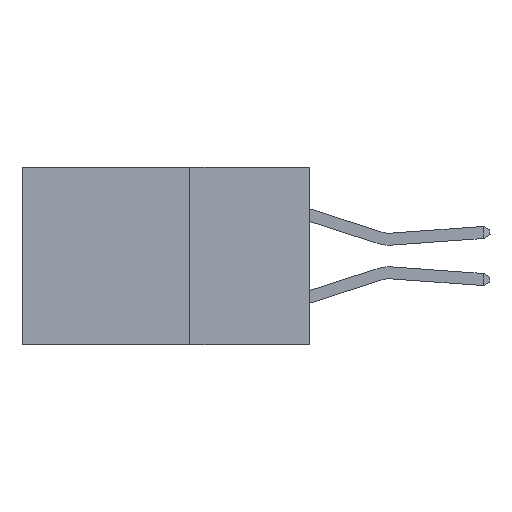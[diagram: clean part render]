
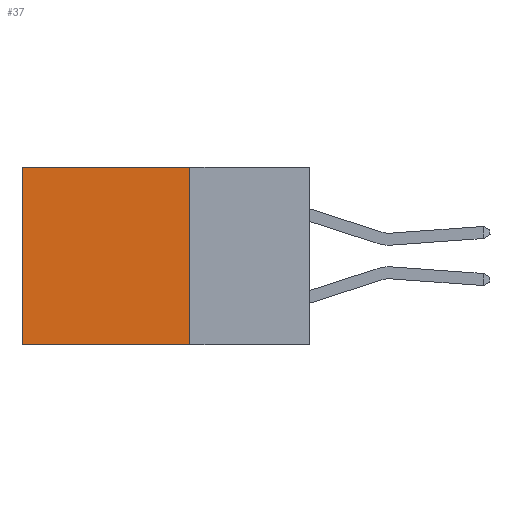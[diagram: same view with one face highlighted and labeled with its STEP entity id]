
A CAD part, left-side view. The second image highlights one B-rep face of the part: STEP entity #37.
In plain terms, the highlighted planar face has unit normal (-1, 0, 0).
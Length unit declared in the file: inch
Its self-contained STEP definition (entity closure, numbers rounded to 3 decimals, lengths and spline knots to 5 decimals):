
#37 = ADVANCED_FACE ( 'NONE', ( #2253 ), #18303, .F. ) ;
#833 = EDGE_LOOP ( 'NONE', ( #8648, #12536, #7388, #7956 ) ) ;
#2059 = LINE ( 'NONE', #13788, #10740 ) ;
#2253 = FACE_OUTER_BOUND ( 'NONE', #833, .T. ) ;
#3085 = DIRECTION ( 'NONE',  ( 0., 0., -1. ) ) ;
#3976 = DIRECTION ( 'NONE',  ( 0., 1., 0. ) ) ;
#4777 = VECTOR ( 'NONE', #19319, 39.37008 ) ;
#6428 = DIRECTION ( 'NONE',  ( 1., 0., 0. ) ) ;
#7052 = EDGE_CURVE ( 'NONE', #10376, #7203, #2059, .T. ) ;
#7203 = VERTEX_POINT ( 'NONE', #9195 ) ;
#7388 = ORIENTED_EDGE ( 'NONE', *, *, #11854, .F. ) ;
#7956 = ORIENTED_EDGE ( 'NONE', *, *, #20057, .T. ) ;
#7968 = DIRECTION ( 'NONE',  ( 0., 0., -1. ) ) ;
#8616 = LINE ( 'NONE', #16102, #16785 ) ;
#8648 = ORIENTED_EDGE ( 'NONE', *, *, #20054, .T. ) ;
#8973 = AXIS2_PLACEMENT_3D ( 'NONE', #20488, #6428, #12057 ) ;
#9195 = CARTESIAN_POINT ( 'NONE',  ( 0.298, 0.6, -0.37 ) ) ;
#10376 = VERTEX_POINT ( 'NONE', #17157 ) ;
#10740 = VECTOR ( 'NONE', #3976, 39.37008 ) ;
#11204 = CARTESIAN_POINT ( 'NONE',  ( 0.298, 0.25, 0. ) ) ;
#11499 = LINE ( 'NONE', #11204, #19573 ) ;
#11854 = EDGE_CURVE ( 'NONE', #19386, #10376, #11499, .T. ) ;
#12057 = DIRECTION ( 'NONE',  ( 0., 0., -1. ) ) ;
#12536 = ORIENTED_EDGE ( 'NONE', *, *, #7052, .F. ) ;
#13246 = CARTESIAN_POINT ( 'NONE',  ( 0.298, 0.6, 0. ) ) ;
#13788 = CARTESIAN_POINT ( 'NONE',  ( 0.298, 0.25, -0.37 ) ) ;
#15849 = CARTESIAN_POINT ( 'NONE',  ( 0.298, 0.25, 0. ) ) ;
#16102 = CARTESIAN_POINT ( 'NONE',  ( 0.298, 0.6, 0. ) ) ;
#16785 = VECTOR ( 'NONE', #7968, 39.37008 ) ;
#17157 = CARTESIAN_POINT ( 'NONE',  ( 0.298, 0.25, -0.37 ) ) ;
#17707 = CARTESIAN_POINT ( 'NONE',  ( 0.298, 0.25, 0. ) ) ;
#18303 = PLANE ( 'NONE',  #8973 ) ;
#19319 = DIRECTION ( 'NONE',  ( 0., 1., 0. ) ) ;
#19386 = VERTEX_POINT ( 'NONE', #15849 ) ;
#19573 = VECTOR ( 'NONE', #3085, 39.37008 ) ;
#20054 = EDGE_CURVE ( 'NONE', #20841, #7203, #8616, .T. ) ;
#20057 = EDGE_CURVE ( 'NONE', #19386, #20841, #21002, .T. ) ;
#20488 = CARTESIAN_POINT ( 'NONE',  ( 0.298, 0.25, 0. ) ) ;
#20841 = VERTEX_POINT ( 'NONE', #13246 ) ;
#21002 = LINE ( 'NONE', #17707, #4777 ) ;
